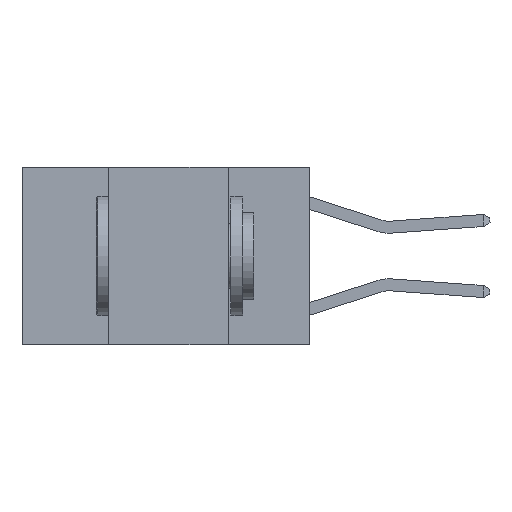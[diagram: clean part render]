
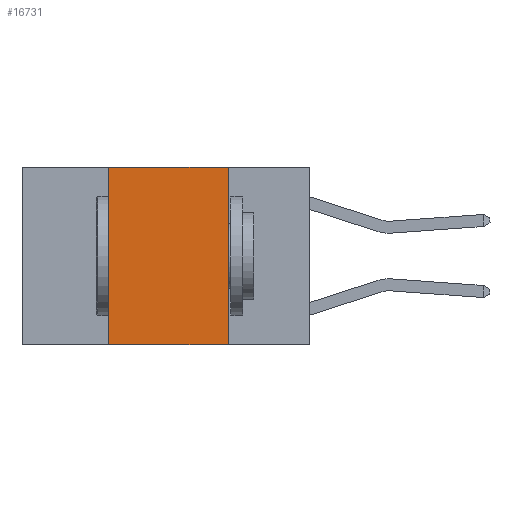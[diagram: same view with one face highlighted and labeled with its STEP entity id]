
A CAD part, left-side view. The second image highlights one B-rep face of the part: STEP entity #16731.
In plain terms, the highlighted planar face has unit normal (-1, 0, 0).
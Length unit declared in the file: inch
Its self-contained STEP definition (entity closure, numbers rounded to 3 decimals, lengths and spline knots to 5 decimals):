
#18 = VECTOR ( 'NONE', #24552, 39.37008 ) ;
#206 = DIRECTION ( 'NONE',  ( 0., 0., -1. ) ) ;
#469 = ORIENTED_EDGE ( 'NONE', *, *, #20973, .F. ) ;
#685 = LINE ( 'NONE', #18653, #5670 ) ;
#952 = VERTEX_POINT ( 'NONE', #17286 ) ;
#1131 = EDGE_CURVE ( 'NONE', #20563, #6965, #23955, .T. ) ;
#2278 = CARTESIAN_POINT ( 'NONE',  ( 0., 0.17, -0.37 ) ) ;
#3366 = CARTESIAN_POINT ( 'NONE',  ( 0., 0.17, 0. ) ) ;
#4387 = VERTEX_POINT ( 'NONE', #2278 ) ;
#5401 = EDGE_CURVE ( 'NONE', #952, #4387, #16936, .T. ) ;
#5627 = DIRECTION ( 'NONE',  ( 0., 0., 1. ) ) ;
#5670 = VECTOR ( 'NONE', #20754, 39.37008 ) ;
#6965 = VERTEX_POINT ( 'NONE', #11480 ) ;
#9105 = EDGE_LOOP ( 'NONE', ( #25464, #469, #14459, #25810 ) ) ;
#10730 = LINE ( 'NONE', #11304, #21944 ) ;
#11304 = CARTESIAN_POINT ( 'NONE',  ( 0., 0.6, 0. ) ) ;
#11480 = CARTESIAN_POINT ( 'NONE',  ( 0., 0.42, 0. ) ) ;
#12810 = PLANE ( 'NONE',  #15818 ) ;
#12894 = DIRECTION ( 'NONE',  ( 1., 0., 0. ) ) ;
#13422 = DIRECTION ( 'NONE',  ( 0., -1., 0. ) ) ;
#14047 = CARTESIAN_POINT ( 'NONE',  ( 0., 0.42, 0. ) ) ;
#14459 = ORIENTED_EDGE ( 'NONE', *, *, #1131, .F. ) ;
#15818 = AXIS2_PLACEMENT_3D ( 'NONE', #25451, #12894, #206 ) ;
#16539 = EDGE_CURVE ( 'NONE', #20563, #4387, #685, .T. ) ;
#16731 = ADVANCED_FACE ( 'NONE', ( #18225 ), #12810, .F. ) ;
#16936 = LINE ( 'NONE', #3366, #18 ) ;
#17286 = CARTESIAN_POINT ( 'NONE',  ( 0., 0.17, 0. ) ) ;
#18225 = FACE_OUTER_BOUND ( 'NONE', #9105, .T. ) ;
#18433 = VECTOR ( 'NONE', #5627, 39.37008 ) ;
#18653 = CARTESIAN_POINT ( 'NONE',  ( 0., 0.6, -0.37 ) ) ;
#20563 = VERTEX_POINT ( 'NONE', #24804 ) ;
#20754 = DIRECTION ( 'NONE',  ( 0., -1., 0. ) ) ;
#20973 = EDGE_CURVE ( 'NONE', #6965, #952, #10730, .T. ) ;
#21944 = VECTOR ( 'NONE', #13422, 39.37008 ) ;
#23955 = LINE ( 'NONE', #14047, #18433 ) ;
#24552 = DIRECTION ( 'NONE',  ( 0., 0., -1. ) ) ;
#24804 = CARTESIAN_POINT ( 'NONE',  ( 0., 0.42, -0.37 ) ) ;
#25451 = CARTESIAN_POINT ( 'NONE',  ( 0., 0.6, 0. ) ) ;
#25464 = ORIENTED_EDGE ( 'NONE', *, *, #5401, .F. ) ;
#25810 = ORIENTED_EDGE ( 'NONE', *, *, #16539, .T. ) ;
